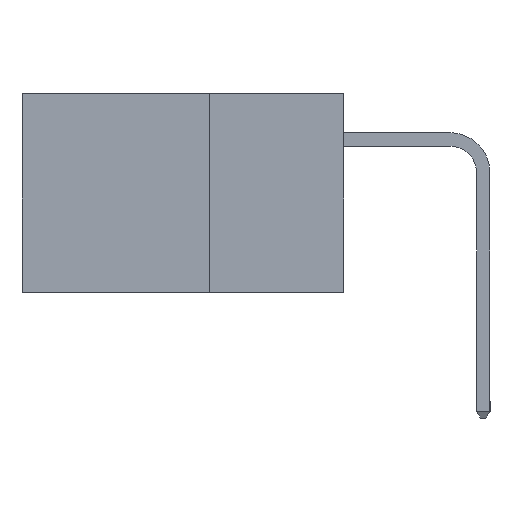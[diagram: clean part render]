
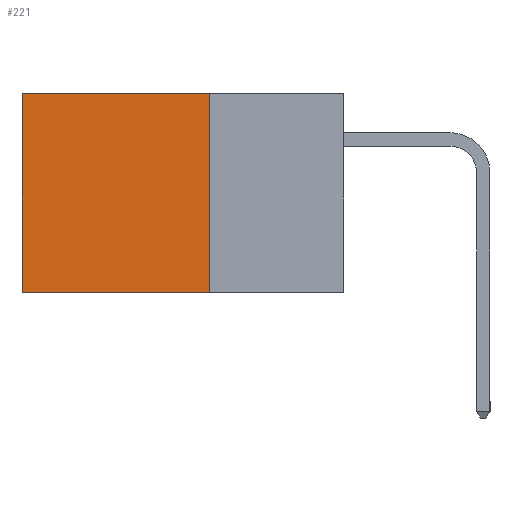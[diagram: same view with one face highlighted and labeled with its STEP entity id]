
A CAD part, left-side view. The second image highlights one B-rep face of the part: STEP entity #221.
In plain terms, the highlighted planar face has unit normal (-1, 0, 0).
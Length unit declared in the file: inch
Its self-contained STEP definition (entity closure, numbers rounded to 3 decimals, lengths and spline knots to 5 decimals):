
#38 = VECTOR ( 'NONE', #11396, 39.37008 ) ;
#221 = ADVANCED_FACE ( 'NONE', ( #5165 ), #2700, .F. ) ;
#1071 = VECTOR ( 'NONE', #9185, 39.37008 ) ;
#1208 = ORIENTED_EDGE ( 'NONE', *, *, #10720, .T. ) ;
#1281 = ORIENTED_EDGE ( 'NONE', *, *, #9130, .F. ) ;
#1321 = ORIENTED_EDGE ( 'NONE', *, *, #2340, .F. ) ;
#1363 = ORIENTED_EDGE ( 'NONE', *, *, #2190, .T. ) ;
#2190 = EDGE_CURVE ( 'NONE', #10636, #11104, #8685, .T. ) ;
#2340 = EDGE_CURVE ( 'NONE', #10636, #3801, #7274, .T. ) ;
#2700 = PLANE ( 'NONE',  #3775 ) ;
#3641 = LINE ( 'NONE', #10010, #1071 ) ;
#3775 = AXIS2_PLACEMENT_3D ( 'NONE', #11479, #6115, #4879 ) ;
#3801 = VERTEX_POINT ( 'NONE', #8850 ) ;
#3826 = CARTESIAN_POINT ( 'NONE',  ( 0.2615, 0.6, -0.37 ) ) ;
#3835 = VECTOR ( 'NONE', #6641, 39.37008 ) ;
#4339 = CARTESIAN_POINT ( 'NONE',  ( 0.2615, 0.6, 0. ) ) ;
#4879 = DIRECTION ( 'NONE',  ( 0., 0., -1. ) ) ;
#5165 = FACE_OUTER_BOUND ( 'NONE', #8437, .T. ) ;
#5917 = CARTESIAN_POINT ( 'NONE',  ( 0.2615, 0.6, -0.37 ) ) ;
#6077 = VERTEX_POINT ( 'NONE', #5917 ) ;
#6115 = DIRECTION ( 'NONE',  ( 1., 0., 0. ) ) ;
#6641 = DIRECTION ( 'NONE',  ( 0., 1., 0. ) ) ;
#6993 = CARTESIAN_POINT ( 'NONE',  ( 0.2615, 0.25, 0. ) ) ;
#7175 = LINE ( 'NONE', #3826, #9552 ) ;
#7274 = LINE ( 'NONE', #11490, #38 ) ;
#8370 = DIRECTION ( 'NONE',  ( 0., 0., -1. ) ) ;
#8437 = EDGE_LOOP ( 'NONE', ( #1208, #1281, #1321, #1363 ) ) ;
#8685 = LINE ( 'NONE', #6993, #3835 ) ;
#8850 = CARTESIAN_POINT ( 'NONE',  ( 0.2615, 0.25, -0.37 ) ) ;
#9120 = CARTESIAN_POINT ( 'NONE',  ( 0.2615, 0.25, 0. ) ) ;
#9130 = EDGE_CURVE ( 'NONE', #3801, #6077, #3641, .T. ) ;
#9185 = DIRECTION ( 'NONE',  ( 0., 1., 0. ) ) ;
#9552 = VECTOR ( 'NONE', #8370, 39.37008 ) ;
#10010 = CARTESIAN_POINT ( 'NONE',  ( 0.2615, 0.25, -0.37 ) ) ;
#10636 = VERTEX_POINT ( 'NONE', #9120 ) ;
#10720 = EDGE_CURVE ( 'NONE', #11104, #6077, #7175, .T. ) ;
#11104 = VERTEX_POINT ( 'NONE', #4339 ) ;
#11396 = DIRECTION ( 'NONE',  ( 0., 0., -1. ) ) ;
#11479 = CARTESIAN_POINT ( 'NONE',  ( 0.2615, 0.25, -0.37 ) ) ;
#11490 = CARTESIAN_POINT ( 'NONE',  ( 0.2615, 0.25, -0.37 ) ) ;
